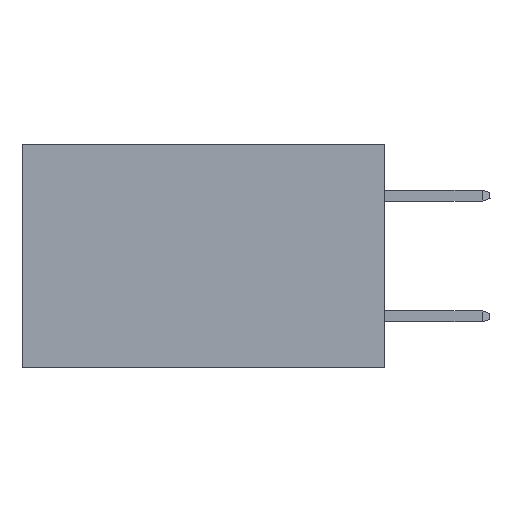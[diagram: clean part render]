
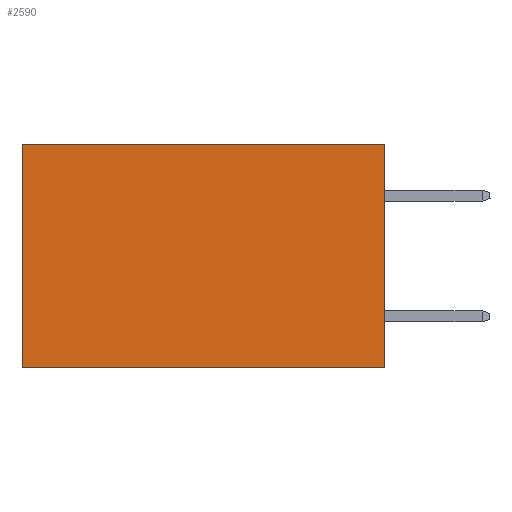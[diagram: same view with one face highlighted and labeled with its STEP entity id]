
A CAD part, left-side view. The second image highlights one B-rep face of the part: STEP entity #2590.
In plain terms, the highlighted planar face has unit normal (-1, 0, 0).
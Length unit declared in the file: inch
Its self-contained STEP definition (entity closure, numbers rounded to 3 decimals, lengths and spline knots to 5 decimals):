
#1683 = EDGE_CURVE ( 'NONE', #5677, #20632, #13231, .T. ) ;
#2251 = VERTEX_POINT ( 'NONE', #4077 ) ;
#2590 = ADVANCED_FACE ( 'NONE', ( #14412 ), #7808, .F. ) ;
#3333 = CARTESIAN_POINT ( 'NONE',  ( 0.298, 0., -0.37 ) ) ;
#3629 = LINE ( 'NONE', #6244, #12201 ) ;
#3661 = LINE ( 'NONE', #3333, #20636 ) ;
#4077 = CARTESIAN_POINT ( 'NONE',  ( 0.298, 0., -0.37 ) ) ;
#4151 = VECTOR ( 'NONE', #13057, 39.37008 ) ;
#4705 = EDGE_LOOP ( 'NONE', ( #13692, #13061, #12471, #6720 ) ) ;
#5523 = CARTESIAN_POINT ( 'NONE',  ( 0.298, 0., 0. ) ) ;
#5677 = VERTEX_POINT ( 'NONE', #11512 ) ;
#5735 = EDGE_CURVE ( 'NONE', #20632, #6007, #3629, .T. ) ;
#6007 = VERTEX_POINT ( 'NONE', #14263 ) ;
#6118 = DIRECTION ( 'NONE',  ( 0., 0., -1. ) ) ;
#6244 = CARTESIAN_POINT ( 'NONE',  ( 0.298, 0.6, 0. ) ) ;
#6720 = ORIENTED_EDGE ( 'NONE', *, *, #1683, .T. ) ;
#7066 = LINE ( 'NONE', #9132, #15584 ) ;
#7808 = PLANE ( 'NONE',  #10903 ) ;
#7824 = CARTESIAN_POINT ( 'NONE',  ( 0.298, 0.6, 0. ) ) ;
#8259 = EDGE_CURVE ( 'NONE', #5677, #2251, #7066, .T. ) ;
#9132 = CARTESIAN_POINT ( 'NONE',  ( 0.298, 0., 0. ) ) ;
#10903 = AXIS2_PLACEMENT_3D ( 'NONE', #14283, #15727, #6118 ) ;
#11512 = CARTESIAN_POINT ( 'NONE',  ( 0.298, 0., 0. ) ) ;
#12201 = VECTOR ( 'NONE', #16427, 39.37008 ) ;
#12471 = ORIENTED_EDGE ( 'NONE', *, *, #8259, .F. ) ;
#13057 = DIRECTION ( 'NONE',  ( 0., 1., 0. ) ) ;
#13061 = ORIENTED_EDGE ( 'NONE', *, *, #16861, .F. ) ;
#13231 = LINE ( 'NONE', #5523, #4151 ) ;
#13692 = ORIENTED_EDGE ( 'NONE', *, *, #5735, .T. ) ;
#14263 = CARTESIAN_POINT ( 'NONE',  ( 0.298, 0.6, -0.37 ) ) ;
#14283 = CARTESIAN_POINT ( 'NONE',  ( 0.298, 0., 0. ) ) ;
#14412 = FACE_OUTER_BOUND ( 'NONE', #4705, .T. ) ;
#14593 = DIRECTION ( 'NONE',  ( 0., 1., 0. ) ) ;
#15584 = VECTOR ( 'NONE', #18700, 39.37008 ) ;
#15727 = DIRECTION ( 'NONE',  ( 1., 0., 0. ) ) ;
#16427 = DIRECTION ( 'NONE',  ( 0., 0., -1. ) ) ;
#16861 = EDGE_CURVE ( 'NONE', #2251, #6007, #3661, .T. ) ;
#18700 = DIRECTION ( 'NONE',  ( 0., 0., -1. ) ) ;
#20632 = VERTEX_POINT ( 'NONE', #7824 ) ;
#20636 = VECTOR ( 'NONE', #14593, 39.37008 ) ;
